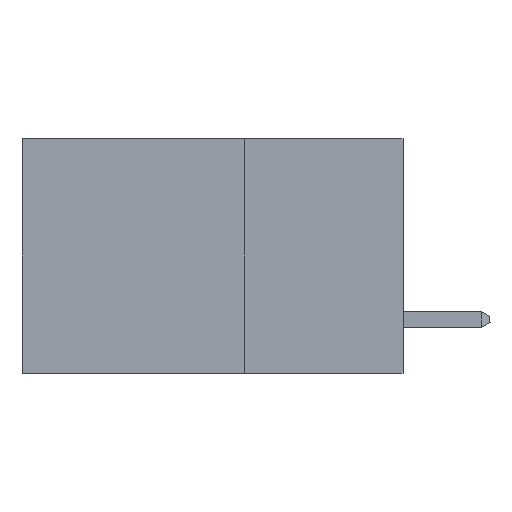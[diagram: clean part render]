
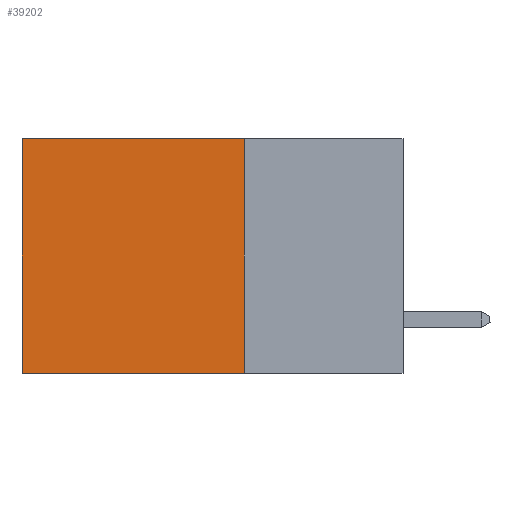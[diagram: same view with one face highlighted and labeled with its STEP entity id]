
A CAD part, left-side view. The second image highlights one B-rep face of the part: STEP entity #39202.
In plain terms, the highlighted planar face has unit normal (-1, 0, 0).
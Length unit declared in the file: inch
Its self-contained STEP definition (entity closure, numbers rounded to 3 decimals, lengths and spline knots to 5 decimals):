
#160 = LINE ( 'NONE', #8664, #20067 ) ;
#1924 = CARTESIAN_POINT ( 'NONE',  ( 0.2875, 0.25, -0.37 ) ) ;
#2933 = CARTESIAN_POINT ( 'NONE',  ( 0.2875, 0.6, 0. ) ) ;
#3832 = ORIENTED_EDGE ( 'NONE', *, *, #6266, .T. ) ;
#4523 = ORIENTED_EDGE ( 'NONE', *, *, #25364, .T. ) ;
#6116 = EDGE_CURVE ( 'NONE', #32085, #34929, #33503, .T. ) ;
#6246 = DIRECTION ( 'NONE',  ( 0., 1., 0. ) ) ;
#6266 = EDGE_CURVE ( 'NONE', #15049, #35823, #14110, .T. ) ;
#6325 = DIRECTION ( 'NONE',  ( 0., 0., -1. ) ) ;
#7465 = VECTOR ( 'NONE', #6325, 39.37008 ) ;
#8664 = CARTESIAN_POINT ( 'NONE',  ( 0.2875, 0.25, 0. ) ) ;
#8970 = CARTESIAN_POINT ( 'NONE',  ( 0.2875, 0.6, 0. ) ) ;
#8978 = CARTESIAN_POINT ( 'NONE',  ( 0.2875, 0.25, 0. ) ) ;
#9033 = ORIENTED_EDGE ( 'NONE', *, *, #36044, .F. ) ;
#13325 = DIRECTION ( 'NONE',  ( 1., 0., 0. ) ) ;
#13741 = FACE_OUTER_BOUND ( 'NONE', #28723, .T. ) ;
#14110 = LINE ( 'NONE', #2933, #7465 ) ;
#15049 = VERTEX_POINT ( 'NONE', #8970 ) ;
#16063 = DIRECTION ( 'NONE',  ( 0., 0., -1. ) ) ;
#16831 = VECTOR ( 'NONE', #6246, 39.37008 ) ;
#17927 = LINE ( 'NONE', #1924, #16831 ) ;
#19970 = DIRECTION ( 'NONE',  ( 0., 0., -1. ) ) ;
#20067 = VECTOR ( 'NONE', #43776, 39.37008 ) ;
#23985 = CARTESIAN_POINT ( 'NONE',  ( 0.2875, 0.25, 0. ) ) ;
#25364 = EDGE_CURVE ( 'NONE', #32085, #15049, #160, .T. ) ;
#27345 = CARTESIAN_POINT ( 'NONE',  ( 0.2875, 0.25, -0.37 ) ) ;
#28723 = EDGE_LOOP ( 'NONE', ( #3832, #9033, #43293, #4523 ) ) ;
#32085 = VERTEX_POINT ( 'NONE', #39556 ) ;
#32392 = VECTOR ( 'NONE', #16063, 39.37008 ) ;
#33503 = LINE ( 'NONE', #8978, #32392 ) ;
#33526 = AXIS2_PLACEMENT_3D ( 'NONE', #23985, #13325, #19970 ) ;
#34929 = VERTEX_POINT ( 'NONE', #27345 ) ;
#35823 = VERTEX_POINT ( 'NONE', #39614 ) ;
#36044 = EDGE_CURVE ( 'NONE', #34929, #35823, #17927, .T. ) ;
#39202 = ADVANCED_FACE ( 'NONE', ( #13741 ), #41615, .F. ) ;
#39556 = CARTESIAN_POINT ( 'NONE',  ( 0.2875, 0.25, 0. ) ) ;
#39614 = CARTESIAN_POINT ( 'NONE',  ( 0.2875, 0.6, -0.37 ) ) ;
#41615 = PLANE ( 'NONE',  #33526 ) ;
#43293 = ORIENTED_EDGE ( 'NONE', *, *, #6116, .F. ) ;
#43776 = DIRECTION ( 'NONE',  ( 0., 1., 0. ) ) ;
